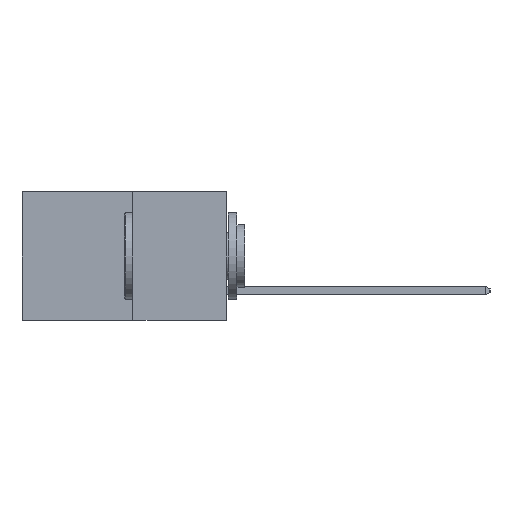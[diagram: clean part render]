
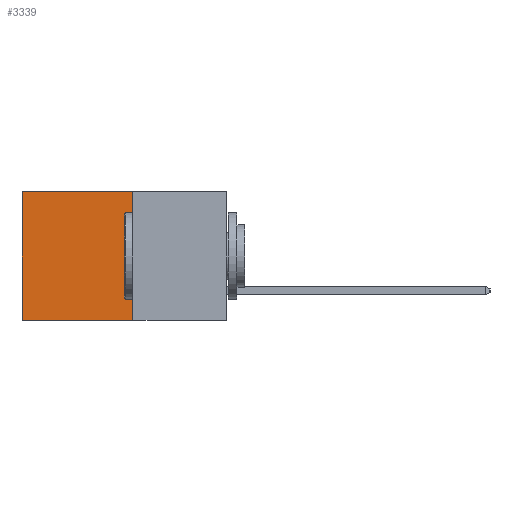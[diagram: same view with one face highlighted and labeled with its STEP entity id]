
A CAD part, left-side view. The second image highlights one B-rep face of the part: STEP entity #3339.
In plain terms, the highlighted planar face has unit normal (-1, 0, 0).
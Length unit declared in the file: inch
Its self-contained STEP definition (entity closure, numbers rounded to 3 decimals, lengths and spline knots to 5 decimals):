
#561 = VERTEX_POINT ( 'NONE', #7403 ) ;
#2159 = ORIENTED_EDGE ( 'NONE', *, *, #20944, .F. ) ;
#3339 = ADVANCED_FACE ( 'NONE', ( #22240 ), #11792, .F. ) ;
#4597 = LINE ( 'NONE', #15228, #21918 ) ;
#5133 = ORIENTED_EDGE ( 'NONE', *, *, #13312, .T. ) ;
#6001 = CARTESIAN_POINT ( 'NONE',  ( 0.277, 0.59, -0.37 ) ) ;
#6136 = CARTESIAN_POINT ( 'NONE',  ( 0.277, 0.27, -0.37 ) ) ;
#7355 = EDGE_LOOP ( 'NONE', ( #7908, #2159, #10228, #5133 ) ) ;
#7403 = CARTESIAN_POINT ( 'NONE',  ( 0.277, 0.27, 0. ) ) ;
#7908 = ORIENTED_EDGE ( 'NONE', *, *, #19719, .T. ) ;
#8255 = EDGE_CURVE ( 'NONE', #561, #14863, #25788, .T. ) ;
#8306 = VERTEX_POINT ( 'NONE', #22127 ) ;
#9900 = CARTESIAN_POINT ( 'NONE',  ( 0.277, 0.27, -0.37 ) ) ;
#10228 = ORIENTED_EDGE ( 'NONE', *, *, #8255, .F. ) ;
#10439 = CARTESIAN_POINT ( 'NONE',  ( 0.277, 0.27, 0. ) ) ;
#10557 = DIRECTION ( 'NONE',  ( 0., 0., -1. ) ) ;
#10592 = DIRECTION ( 'NONE',  ( 1., 0., 0. ) ) ;
#11718 = AXIS2_PLACEMENT_3D ( 'NONE', #11753, #10592, #10557 ) ;
#11753 = CARTESIAN_POINT ( 'NONE',  ( 0.277, 0.27, -0.37 ) ) ;
#11792 = PLANE ( 'NONE',  #11718 ) ;
#13312 = EDGE_CURVE ( 'NONE', #561, #8306, #15486, .T. ) ;
#14863 = VERTEX_POINT ( 'NONE', #26768 ) ;
#14935 = DIRECTION ( 'NONE',  ( 0., 1., 0. ) ) ;
#15154 = DIRECTION ( 'NONE',  ( 0., 0., -1. ) ) ;
#15228 = CARTESIAN_POINT ( 'NONE',  ( 0.277, 0.59, -0.37 ) ) ;
#15486 = LINE ( 'NONE', #10439, #26754 ) ;
#17542 = DIRECTION ( 'NONE',  ( 0., 0., -1. ) ) ;
#19719 = EDGE_CURVE ( 'NONE', #8306, #26309, #4597, .T. ) ;
#19829 = VECTOR ( 'NONE', #15154, 39.37008 ) ;
#20457 = VECTOR ( 'NONE', #27854, 39.37008 ) ;
#20944 = EDGE_CURVE ( 'NONE', #14863, #26309, #25690, .T. ) ;
#21918 = VECTOR ( 'NONE', #17542, 39.37008 ) ;
#22127 = CARTESIAN_POINT ( 'NONE',  ( 0.277, 0.59, 0. ) ) ;
#22240 = FACE_OUTER_BOUND ( 'NONE', #7355, .T. ) ;
#25690 = LINE ( 'NONE', #9900, #20457 ) ;
#25788 = LINE ( 'NONE', #6136, #19829 ) ;
#26309 = VERTEX_POINT ( 'NONE', #6001 ) ;
#26754 = VECTOR ( 'NONE', #14935, 39.37008 ) ;
#26768 = CARTESIAN_POINT ( 'NONE',  ( 0.277, 0.27, -0.37 ) ) ;
#27854 = DIRECTION ( 'NONE',  ( 0., 1., 0. ) ) ;
